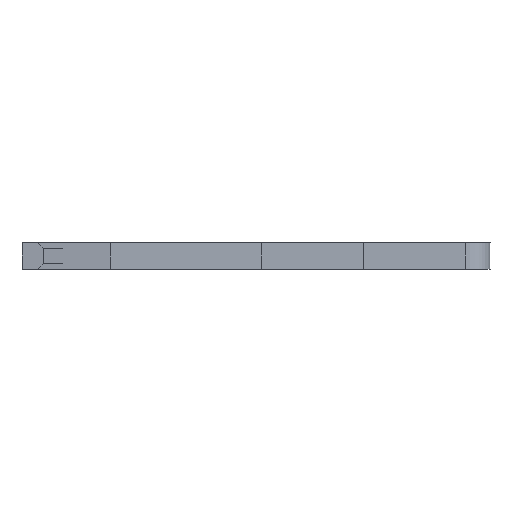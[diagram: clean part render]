
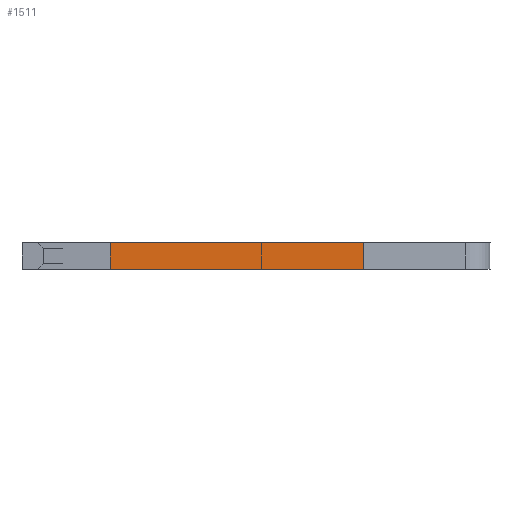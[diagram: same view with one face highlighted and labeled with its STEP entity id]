
A CAD part, left-side view. The second image highlights one B-rep face of the part: STEP entity #1511.
In plain terms, the highlighted face is planar.
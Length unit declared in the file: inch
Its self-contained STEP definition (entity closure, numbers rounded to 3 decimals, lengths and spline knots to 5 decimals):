
#85 = CARTESIAN_POINT ( 'NONE',  ( 0.013, 0.146, -0.0575 ) ) ;
#129 = CARTESIAN_POINT ( 'NONE',  ( 0.013, -0.099, -0.0575 ) ) ;
#209 = ORIENTED_EDGE ( 'NONE', *, *, #234, .F. ) ;
#217 = PLANE ( 'NONE',  #993 ) ;
#234 = EDGE_CURVE ( 'NONE', #934, #2296, #678, .T. ) ;
#240 = DIRECTION ( 'NONE',  ( 1., 0., 0. ) ) ;
#261 = DIRECTION ( 'NONE',  ( 0., 1., 0. ) ) ;
#342 = CARTESIAN_POINT ( 'NONE',  ( -0.013, 0.146, -0.0575 ) ) ;
#374 = ORIENTED_EDGE ( 'NONE', *, *, #1733, .T. ) ;
#404 = LINE ( 'NONE', #2019, #922 ) ;
#582 = ORIENTED_EDGE ( 'NONE', *, *, #1790, .F. ) ;
#654 = CARTESIAN_POINT ( 'NONE',  ( 0.013, 0.146, -0.0575 ) ) ;
#678 = LINE ( 'NONE', #937, #2562 ) ;
#922 = VECTOR ( 'NONE', #1370, 39.37008 ) ;
#934 = VERTEX_POINT ( 'NONE', #129 ) ;
#937 = CARTESIAN_POINT ( 'NONE',  ( 0.013, 0.146, -0.0575 ) ) ;
#986 = LINE ( 'NONE', #1895, #2727 ) ;
#993 = AXIS2_PLACEMENT_3D ( 'NONE', #654, #2180, #240 ) ;
#1107 = CARTESIAN_POINT ( 'NONE',  ( 0.013, -0.099, -0.0575 ) ) ;
#1118 = VECTOR ( 'NONE', #2645, 39.37008 ) ;
#1230 = DIRECTION ( 'NONE',  ( 0., 1., 0. ) ) ;
#1370 = DIRECTION ( 'NONE',  ( -1., 0., 0. ) ) ;
#1511 = ADVANCED_FACE ( 'NONE', ( #2696 ), #217, .F. ) ;
#1533 = LINE ( 'NONE', #1107, #1118 ) ;
#1550 = ORIENTED_EDGE ( 'NONE', *, *, #2742, .T. ) ;
#1733 = EDGE_CURVE ( 'NONE', #934, #2497, #1533, .T. ) ;
#1790 = EDGE_CURVE ( 'NONE', #2296, #2734, #404, .T. ) ;
#1895 = CARTESIAN_POINT ( 'NONE',  ( -0.013, 0.146, -0.0575 ) ) ;
#2019 = CARTESIAN_POINT ( 'NONE',  ( 0.013, 0.146, -0.0575 ) ) ;
#2089 = CARTESIAN_POINT ( 'NONE',  ( -0.013, -0.099, -0.0575 ) ) ;
#2180 = DIRECTION ( 'NONE',  ( 0., 0., 1. ) ) ;
#2220 = EDGE_LOOP ( 'NONE', ( #1550, #582, #209, #374 ) ) ;
#2296 = VERTEX_POINT ( 'NONE', #85 ) ;
#2497 = VERTEX_POINT ( 'NONE', #2089 ) ;
#2562 = VECTOR ( 'NONE', #261, 39.37008 ) ;
#2645 = DIRECTION ( 'NONE',  ( -1., 0., 0. ) ) ;
#2696 = FACE_OUTER_BOUND ( 'NONE', #2220, .T. ) ;
#2727 = VECTOR ( 'NONE', #1230, 39.37008 ) ;
#2734 = VERTEX_POINT ( 'NONE', #342 ) ;
#2742 = EDGE_CURVE ( 'NONE', #2497, #2734, #986, .T. ) ;
